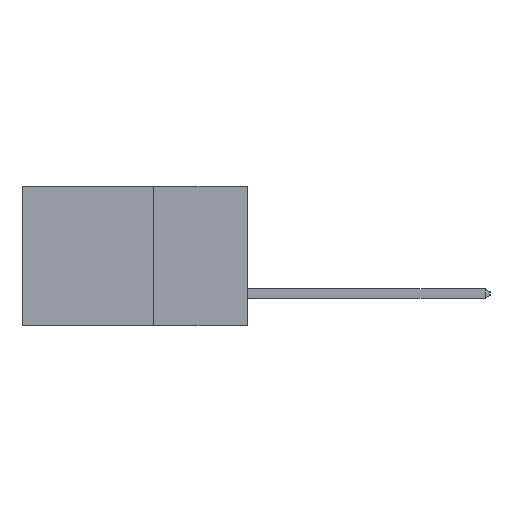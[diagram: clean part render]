
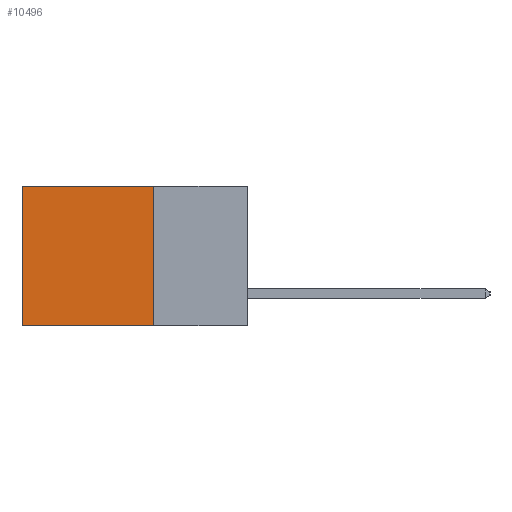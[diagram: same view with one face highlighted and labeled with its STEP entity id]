
A CAD part, left-side view. The second image highlights one B-rep face of the part: STEP entity #10496.
In plain terms, the highlighted planar face has unit normal (-1, 0, 0).
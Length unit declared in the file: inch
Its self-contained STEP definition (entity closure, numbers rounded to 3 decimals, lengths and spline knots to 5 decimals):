
#338 = LINE ( 'NONE', #11824, #5179 ) ;
#763 = DIRECTION ( 'NONE',  ( 1., 0., 0. ) ) ;
#852 = EDGE_CURVE ( 'NONE', #12201, #6399, #3921, .T. ) ;
#1558 = VECTOR ( 'NONE', #6174, 39.37008 ) ;
#1806 = VERTEX_POINT ( 'NONE', #4614 ) ;
#2987 = VECTOR ( 'NONE', #5418, 39.37008 ) ;
#3102 = ORIENTED_EDGE ( 'NONE', *, *, #11531, .F. ) ;
#3921 = LINE ( 'NONE', #6192, #1558 ) ;
#4478 = DIRECTION ( 'NONE',  ( 0., 1., 0. ) ) ;
#4614 = CARTESIAN_POINT ( 'NONE',  ( 0.298, 0.25, 0. ) ) ;
#4963 = DIRECTION ( 'NONE',  ( 0., 1., 0. ) ) ;
#5179 = VECTOR ( 'NONE', #4478, 39.37008 ) ;
#5289 = VERTEX_POINT ( 'NONE', #12746 ) ;
#5418 = DIRECTION ( 'NONE',  ( 0., 0., -1. ) ) ;
#5666 = FACE_OUTER_BOUND ( 'NONE', #11827, .T. ) ;
#6174 = DIRECTION ( 'NONE',  ( 0., 0., -1. ) ) ;
#6192 = CARTESIAN_POINT ( 'NONE',  ( 0.298, 0.6, 0. ) ) ;
#6399 = VERTEX_POINT ( 'NONE', #12463 ) ;
#6916 = ORIENTED_EDGE ( 'NONE', *, *, #10247, .T. ) ;
#6928 = EDGE_CURVE ( 'NONE', #5289, #6399, #8517, .T. ) ;
#6961 = PLANE ( 'NONE',  #11857 ) ;
#8013 = DIRECTION ( 'NONE',  ( 0., 0., -1. ) ) ;
#8517 = LINE ( 'NONE', #12271, #13333 ) ;
#8583 = LINE ( 'NONE', #11648, #2987 ) ;
#9620 = CARTESIAN_POINT ( 'NONE',  ( 0.298, 0.6, 0. ) ) ;
#9682 = ORIENTED_EDGE ( 'NONE', *, *, #6928, .F. ) ;
#10247 = EDGE_CURVE ( 'NONE', #1806, #12201, #338, .T. ) ;
#10496 = ADVANCED_FACE ( 'NONE', ( #5666 ), #6961, .F. ) ;
#11531 = EDGE_CURVE ( 'NONE', #1806, #5289, #8583, .T. ) ;
#11648 = CARTESIAN_POINT ( 'NONE',  ( 0.298, 0.25, 0. ) ) ;
#11824 = CARTESIAN_POINT ( 'NONE',  ( 0.298, 0.25, 0. ) ) ;
#11827 = EDGE_LOOP ( 'NONE', ( #12987, #9682, #3102, #6916 ) ) ;
#11857 = AXIS2_PLACEMENT_3D ( 'NONE', #12166, #763, #8013 ) ;
#12166 = CARTESIAN_POINT ( 'NONE',  ( 0.298, 0.25, 0. ) ) ;
#12201 = VERTEX_POINT ( 'NONE', #9620 ) ;
#12271 = CARTESIAN_POINT ( 'NONE',  ( 0.298, 0.25, -0.37 ) ) ;
#12463 = CARTESIAN_POINT ( 'NONE',  ( 0.298, 0.6, -0.37 ) ) ;
#12746 = CARTESIAN_POINT ( 'NONE',  ( 0.298, 0.25, -0.37 ) ) ;
#12987 = ORIENTED_EDGE ( 'NONE', *, *, #852, .T. ) ;
#13333 = VECTOR ( 'NONE', #4963, 39.37008 ) ;
